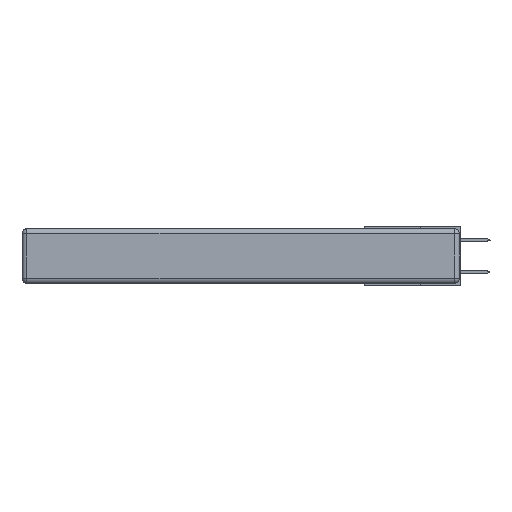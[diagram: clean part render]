
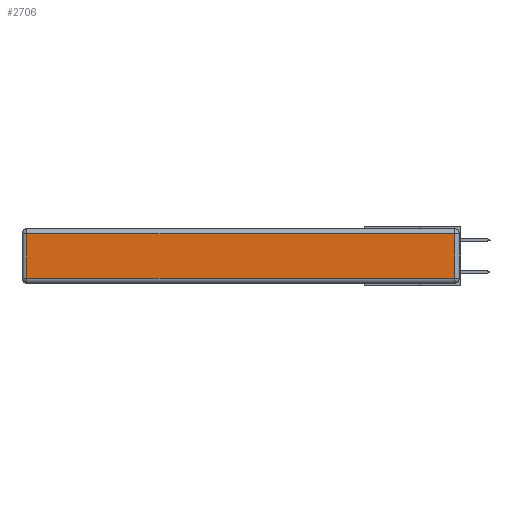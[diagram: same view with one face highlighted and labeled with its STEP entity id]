
A CAD part, left-side view. The second image highlights one B-rep face of the part: STEP entity #2706.
In plain terms, the highlighted planar face has unit normal (-1, 0, 0).
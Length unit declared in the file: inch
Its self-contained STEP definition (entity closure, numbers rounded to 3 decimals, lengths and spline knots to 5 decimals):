
#836 = FACE_OUTER_BOUND ( 'NONE', #17196, .T. ) ;
#912 = CARTESIAN_POINT ( 'NONE',  ( 0., 2.72, -0.03 ) ) ;
#1122 = AXIS2_PLACEMENT_3D ( 'NONE', #9628, #5410, #25766 ) ;
#2075 = CARTESIAN_POINT ( 'NONE',  ( 0., 0.03, -0.313 ) ) ;
#2706 = ADVANCED_FACE ( 'NONE', ( #836 ), #26024, .T. ) ;
#4152 = DIRECTION ( 'NONE',  ( 0., 0., -1. ) ) ;
#4415 = ORIENTED_EDGE ( 'NONE', *, *, #16349, .T. ) ;
#4981 = VERTEX_POINT ( 'NONE', #912 ) ;
#5410 = DIRECTION ( 'NONE',  ( -1., 0., 0. ) ) ;
#6089 = LINE ( 'NONE', #17706, #17000 ) ;
#7150 = CARTESIAN_POINT ( 'NONE',  ( 0., 0.03, -0.03 ) ) ;
#7151 = VERTEX_POINT ( 'NONE', #2075 ) ;
#7387 = LINE ( 'NONE', #16109, #9921 ) ;
#8032 = DIRECTION ( 'NONE',  ( 0., 0., 1. ) ) ;
#9628 = CARTESIAN_POINT ( 'NONE',  ( 0., 0., -0.343 ) ) ;
#9921 = VECTOR ( 'NONE', #22288, 39.37008 ) ;
#12281 = CARTESIAN_POINT ( 'NONE',  ( 0., 2.72, -0.313 ) ) ;
#12553 = CARTESIAN_POINT ( 'NONE',  ( 0., 2.72, -0.343 ) ) ;
#12906 = ORIENTED_EDGE ( 'NONE', *, *, #25225, .T. ) ;
#13181 = VERTEX_POINT ( 'NONE', #7150 ) ;
#13575 = ORIENTED_EDGE ( 'NONE', *, *, #20554, .T. ) ;
#16109 = CARTESIAN_POINT ( 'NONE',  ( 0., 2.75, -0.03 ) ) ;
#16349 = EDGE_CURVE ( 'NONE', #16543, #7151, #16582, .T. ) ;
#16543 = VERTEX_POINT ( 'NONE', #12281 ) ;
#16582 = LINE ( 'NONE', #25080, #17534 ) ;
#17000 = VECTOR ( 'NONE', #8032, 39.37008 ) ;
#17196 = EDGE_LOOP ( 'NONE', ( #4415, #12906, #19143, #13575 ) ) ;
#17534 = VECTOR ( 'NONE', #20881, 39.37008 ) ;
#17706 = CARTESIAN_POINT ( 'NONE',  ( 0., 0.03, -0.343 ) ) ;
#19143 = ORIENTED_EDGE ( 'NONE', *, *, #22527, .T. ) ;
#20554 = EDGE_CURVE ( 'NONE', #4981, #16543, #24072, .T. ) ;
#20881 = DIRECTION ( 'NONE',  ( 0., -1., 0. ) ) ;
#22288 = DIRECTION ( 'NONE',  ( 0., 1., 0. ) ) ;
#22527 = EDGE_CURVE ( 'NONE', #13181, #4981, #7387, .T. ) ;
#22778 = VECTOR ( 'NONE', #4152, 39.37008 ) ;
#24072 = LINE ( 'NONE', #12553, #22778 ) ;
#25080 = CARTESIAN_POINT ( 'NONE',  ( 0., 0., -0.313 ) ) ;
#25225 = EDGE_CURVE ( 'NONE', #7151, #13181, #6089, .T. ) ;
#25766 = DIRECTION ( 'NONE',  ( 0., 0., 1. ) ) ;
#26024 = PLANE ( 'NONE',  #1122 ) ;
